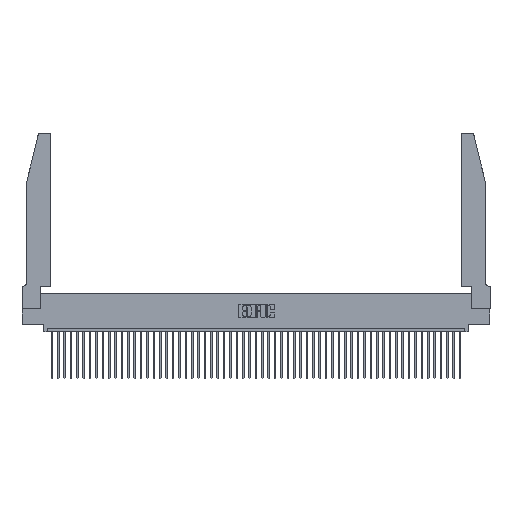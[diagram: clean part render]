
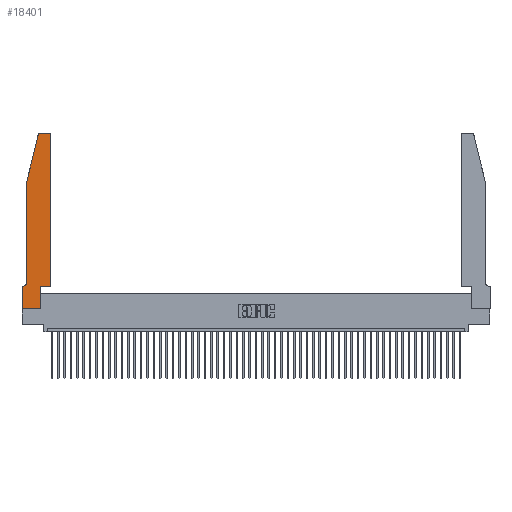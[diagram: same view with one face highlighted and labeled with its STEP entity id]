
A CAD part, top view. The second image highlights one B-rep face of the part: STEP entity #18401.
In plain terms, the highlighted planar face has unit normal (0, 0, 1).
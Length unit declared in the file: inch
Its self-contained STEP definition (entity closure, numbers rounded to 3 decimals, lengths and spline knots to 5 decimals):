
#391 = LINE ( 'NONE', #19419, #34761 ) ;
#1154 = VERTEX_POINT ( 'NONE', #29316 ) ;
#1177 = EDGE_CURVE ( 'NONE', #50486, #36432, #7658, .T. ) ;
#1703 = DIRECTION ( 'NONE',  ( 1., 0., 0. ) ) ;
#1833 = VERTEX_POINT ( 'NONE', #16074 ) ;
#2427 = DIRECTION ( 'NONE',  ( 1., 0., 0. ) ) ;
#2768 = LINE ( 'NONE', #11972, #8138 ) ;
#3282 = AXIS2_PLACEMENT_3D ( 'NONE', #31578, #27836, #8289 ) ;
#3420 = DIRECTION ( 'NONE',  ( 0., -1., 0. ) ) ;
#5002 = PLANE ( 'NONE',  #31372 ) ;
#5536 = LINE ( 'NONE', #9696, #46005 ) ;
#6854 = DIRECTION ( 'NONE',  ( 0., 0., 1. ) ) ;
#7337 = DIRECTION ( 'NONE',  ( 1., 0., 0. ) ) ;
#7400 = VECTOR ( 'NONE', #33829, 39.37008 ) ;
#7658 = LINE ( 'NONE', #33581, #37685 ) ;
#8138 = VECTOR ( 'NONE', #34916, 39.37008 ) ;
#8289 = DIRECTION ( 'NONE',  ( -1., 0., 0. ) ) ;
#8407 = AXIS2_PLACEMENT_3D ( 'NONE', #16959, #32699, #1703 ) ;
#8455 = CARTESIAN_POINT ( 'NONE',  ( 0., 0.35, 0.37 ) ) ;
#9553 = EDGE_CURVE ( 'NONE', #22693, #32668, #46616, .T. ) ;
#9696 = CARTESIAN_POINT ( 'NONE',  ( 0.0755, 0.35, 0.37 ) ) ;
#11862 = ORIENTED_EDGE ( 'NONE', *, *, #45499, .T. ) ;
#11908 = CARTESIAN_POINT ( 'NONE',  ( 0., 0., 0.37 ) ) ;
#11967 = ORIENTED_EDGE ( 'NONE', *, *, #1177, .T. ) ;
#11972 = CARTESIAN_POINT ( 'NONE',  ( 0.4505, 0.35, 0.37 ) ) ;
#13137 = CARTESIAN_POINT ( 'NONE',  ( 0.2865, 0.35, 0.37 ) ) ;
#14186 = EDGE_CURVE ( 'NONE', #41128, #22693, #2768, .T. ) ;
#15468 = DIRECTION ( 'NONE',  ( -0.239, -0.971, 0. ) ) ;
#15781 = EDGE_CURVE ( 'NONE', #19356, #41128, #391, .T. ) ;
#16074 = CARTESIAN_POINT ( 'NONE',  ( 0.0755, 2., 0.37 ) ) ;
#16819 = ORIENTED_EDGE ( 'NONE', *, *, #45536, .T. ) ;
#16861 = VECTOR ( 'NONE', #20650, 39.37008 ) ;
#16959 = CARTESIAN_POINT ( 'NONE',  ( 0.4205, 2.72, 0.37 ) ) ;
#17851 = LINE ( 'NONE', #49568, #50271 ) ;
#17915 = ORIENTED_EDGE ( 'NONE', *, *, #19190, .T. ) ;
#17965 = CIRCLE ( 'NONE', #8407, 0.03 ) ;
#18006 = VECTOR ( 'NONE', #15468, 39.37008 ) ;
#18401 = ADVANCED_FACE ( 'NONE', ( #28405 ), #5002, .T. ) ;
#19190 = EDGE_CURVE ( 'NONE', #32668, #40609, #17965, .T. ) ;
#19341 = EDGE_CURVE ( 'NONE', #40609, #1154, #38700, .T. ) ;
#19356 = VERTEX_POINT ( 'NONE', #43741 ) ;
#19419 = CARTESIAN_POINT ( 'NONE',  ( 0.2865, 0.35, 0.37 ) ) ;
#19856 = CARTESIAN_POINT ( 'NONE',  ( 0.2605, 2.75, 0.37 ) ) ;
#20650 = DIRECTION ( 'NONE',  ( 1., 0., 0. ) ) ;
#20689 = ORIENTED_EDGE ( 'NONE', *, *, #14186, .T. ) ;
#20938 = ORIENTED_EDGE ( 'NONE', *, *, #25382, .T. ) ;
#22368 = LINE ( 'NONE', #23864, #18006 ) ;
#22693 = VERTEX_POINT ( 'NONE', #39790 ) ;
#23631 = ORIENTED_EDGE ( 'NONE', *, *, #45846, .T. ) ;
#23864 = CARTESIAN_POINT ( 'NONE',  ( 0.0755, 2., 0.37 ) ) ;
#24436 = VERTEX_POINT ( 'NONE', #39183 ) ;
#25382 = EDGE_CURVE ( 'NONE', #36432, #19356, #49329, .T. ) ;
#25718 = VERTEX_POINT ( 'NONE', #36268 ) ;
#25816 = CARTESIAN_POINT ( 'NONE',  ( 0.4505, 2.72, 0.37 ) ) ;
#26563 = ORIENTED_EDGE ( 'NONE', *, *, #45193, .T. ) ;
#26601 = ORIENTED_EDGE ( 'NONE', *, *, #15781, .T. ) ;
#27836 = DIRECTION ( 'NONE',  ( 0., 0., -1. ) ) ;
#28405 = FACE_OUTER_BOUND ( 'NONE', #31520, .T. ) ;
#29316 = CARTESIAN_POINT ( 'NONE',  ( 0.284, 2.75, 0.37 ) ) ;
#29666 = CARTESIAN_POINT ( 'NONE',  ( 0.4205, 2.75, 0.37 ) ) ;
#31372 = AXIS2_PLACEMENT_3D ( 'NONE', #50160, #6854, #7337 ) ;
#31520 = EDGE_LOOP ( 'NONE', ( #40427, #46701, #23631, #16819, #26563, #11862, #11967, #20938, #26601, #20689, #49961, #17915 ) ) ;
#31578 = CARTESIAN_POINT ( 'NONE',  ( 0.0055, 0.42, 0.37 ) ) ;
#31642 = DIRECTION ( 'NONE',  ( -1., 0., 0. ) ) ;
#32668 = VERTEX_POINT ( 'NONE', #25816 ) ;
#32699 = DIRECTION ( 'NONE',  ( 0., 0., 1. ) ) ;
#33179 = CIRCLE ( 'NONE', #3282, 0.07 ) ;
#33581 = CARTESIAN_POINT ( 'NONE',  ( 0., 0., 0.37 ) ) ;
#33586 = CARTESIAN_POINT ( 'NONE',  ( 0., 0., 0.37 ) ) ;
#33829 = DIRECTION ( 'NONE',  ( 0., 1., 0. ) ) ;
#34761 = VECTOR ( 'NONE', #50229, 39.37008 ) ;
#34916 = DIRECTION ( 'NONE',  ( 1., 0., 0. ) ) ;
#36228 = VECTOR ( 'NONE', #31642, 39.37008 ) ;
#36268 = CARTESIAN_POINT ( 'NONE',  ( 0.25487, 2.72718, 0.37 ) ) ;
#36432 = VERTEX_POINT ( 'NONE', #33586 ) ;
#36980 = CARTESIAN_POINT ( 'NONE',  ( 0.0755, 0.42, 0.37 ) ) ;
#37209 = DIRECTION ( 'NONE',  ( 0., -1., 0. ) ) ;
#37627 = CARTESIAN_POINT ( 'NONE',  ( 0.284, 2.72, 0.37 ) ) ;
#37685 = VECTOR ( 'NONE', #3420, 39.37008 ) ;
#38700 = LINE ( 'NONE', #19856, #36228 ) ;
#39183 = CARTESIAN_POINT ( 'NONE',  ( 0.0055, 0.35, 0.37 ) ) ;
#39790 = CARTESIAN_POINT ( 'NONE',  ( 0.4505, 0.35, 0.37 ) ) ;
#40427 = ORIENTED_EDGE ( 'NONE', *, *, #19341, .T. ) ;
#40609 = VERTEX_POINT ( 'NONE', #29666 ) ;
#40982 = DIRECTION ( 'NONE',  ( -1., 0., 0. ) ) ;
#41128 = VERTEX_POINT ( 'NONE', #13137 ) ;
#42422 = AXIS2_PLACEMENT_3D ( 'NONE', #37627, #49301, #2427 ) ;
#43741 = CARTESIAN_POINT ( 'NONE',  ( 0.2865, 0., 0.37 ) ) ;
#45193 = EDGE_CURVE ( 'NONE', #49477, #24436, #33179, .T. ) ;
#45499 = EDGE_CURVE ( 'NONE', #24436, #50486, #5536, .T. ) ;
#45536 = EDGE_CURVE ( 'NONE', #1833, #49477, #17851, .T. ) ;
#45846 = EDGE_CURVE ( 'NONE', #25718, #1833, #22368, .T. ) ;
#45901 = CIRCLE ( 'NONE', #42422, 0.03 ) ;
#45960 = CARTESIAN_POINT ( 'NONE',  ( 0.4505, 0.35, 0.37 ) ) ;
#46005 = VECTOR ( 'NONE', #40982, 39.37008 ) ;
#46616 = LINE ( 'NONE', #45960, #7400 ) ;
#46701 = ORIENTED_EDGE ( 'NONE', *, *, #47276, .T. ) ;
#47276 = EDGE_CURVE ( 'NONE', #1154, #25718, #45901, .T. ) ;
#49301 = DIRECTION ( 'NONE',  ( 0., 0., 1. ) ) ;
#49329 = LINE ( 'NONE', #11908, #16861 ) ;
#49477 = VERTEX_POINT ( 'NONE', #36980 ) ;
#49568 = CARTESIAN_POINT ( 'NONE',  ( 0.0755, 2., 0.37 ) ) ;
#49961 = ORIENTED_EDGE ( 'NONE', *, *, #9553, .T. ) ;
#50160 = CARTESIAN_POINT ( 'NONE',  ( 0., 0.35, 0.37 ) ) ;
#50229 = DIRECTION ( 'NONE',  ( 0., 1., 0. ) ) ;
#50271 = VECTOR ( 'NONE', #37209, 39.37008 ) ;
#50486 = VERTEX_POINT ( 'NONE', #8455 ) ;
